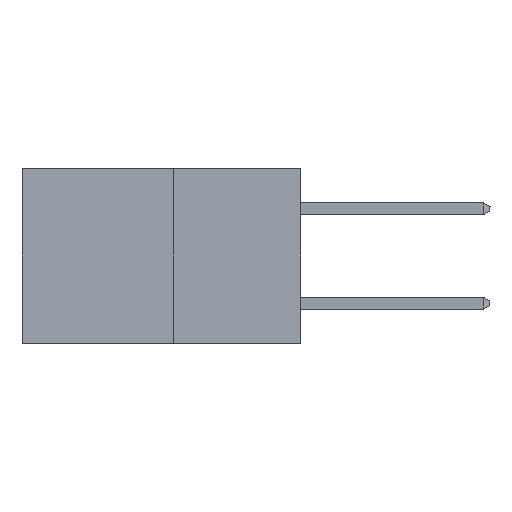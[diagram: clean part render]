
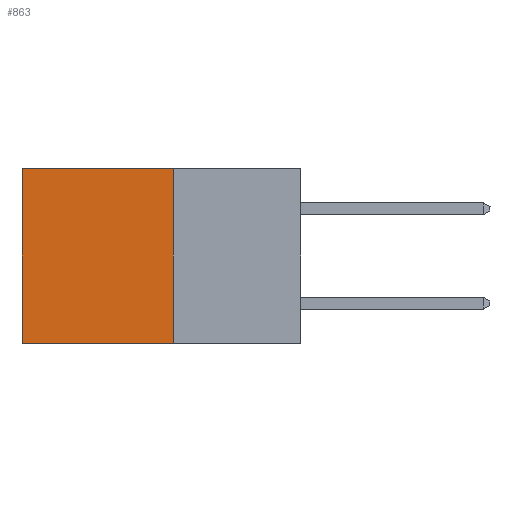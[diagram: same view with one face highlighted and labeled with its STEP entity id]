
A CAD part, left-side view. The second image highlights one B-rep face of the part: STEP entity #863.
In plain terms, the highlighted planar face has unit normal (-1, 0, 0).
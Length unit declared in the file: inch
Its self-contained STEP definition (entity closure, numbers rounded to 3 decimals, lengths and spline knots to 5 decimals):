
#84 = PLANE ( 'NONE',  #2871 ) ;
#150 = EDGE_CURVE ( 'NONE', #2724, #8112, #6001, .T. ) ;
#863 = ADVANCED_FACE ( 'NONE', ( #5290 ), #84, .F. ) ;
#902 = EDGE_CURVE ( 'NONE', #10497, #6457, #2334, .T. ) ;
#979 = ORIENTED_EDGE ( 'NONE', *, *, #902, .T. ) ;
#1040 = DIRECTION ( 'NONE',  ( 0., 0., -1. ) ) ;
#1282 = CARTESIAN_POINT ( 'NONE',  ( 0.277, 0.27, 0. ) ) ;
#2030 = EDGE_LOOP ( 'NONE', ( #979, #2833, #5757, #5247 ) ) ;
#2334 = LINE ( 'NONE', #10953, #6819 ) ;
#2363 = EDGE_CURVE ( 'NONE', #8112, #6457, #9028, .T. ) ;
#2724 = VERTEX_POINT ( 'NONE', #1282 ) ;
#2833 = ORIENTED_EDGE ( 'NONE', *, *, #2363, .F. ) ;
#2871 = AXIS2_PLACEMENT_3D ( 'NONE', #8211, #6450, #1040 ) ;
#3602 = EDGE_CURVE ( 'NONE', #2724, #10497, #7363, .T. ) ;
#3968 = CARTESIAN_POINT ( 'NONE',  ( 0.277, 0.27, -0.37 ) ) ;
#5178 = CARTESIAN_POINT ( 'NONE',  ( 0.277, 0.27, -0.37 ) ) ;
#5247 = ORIENTED_EDGE ( 'NONE', *, *, #3602, .T. ) ;
#5290 = FACE_OUTER_BOUND ( 'NONE', #2030, .T. ) ;
#5425 = CARTESIAN_POINT ( 'NONE',  ( 0.277, 0.27, -0.37 ) ) ;
#5757 = ORIENTED_EDGE ( 'NONE', *, *, #150, .F. ) ;
#6001 = LINE ( 'NONE', #3968, #7861 ) ;
#6045 = CARTESIAN_POINT ( 'NONE',  ( 0.277, 0.27, 0. ) ) ;
#6450 = DIRECTION ( 'NONE',  ( 1., 0., 0. ) ) ;
#6457 = VERTEX_POINT ( 'NONE', #6774 ) ;
#6608 = DIRECTION ( 'NONE',  ( 0., 0., -1. ) ) ;
#6637 = VECTOR ( 'NONE', #7957, 39.37008 ) ;
#6774 = CARTESIAN_POINT ( 'NONE',  ( 0.277, 0.59, -0.37 ) ) ;
#6819 = VECTOR ( 'NONE', #7472, 39.37008 ) ;
#7363 = LINE ( 'NONE', #6045, #9687 ) ;
#7472 = DIRECTION ( 'NONE',  ( 0., 0., -1. ) ) ;
#7861 = VECTOR ( 'NONE', #6608, 39.37008 ) ;
#7957 = DIRECTION ( 'NONE',  ( 0., 1., 0. ) ) ;
#8112 = VERTEX_POINT ( 'NONE', #5425 ) ;
#8211 = CARTESIAN_POINT ( 'NONE',  ( 0.277, 0.27, -0.37 ) ) ;
#9028 = LINE ( 'NONE', #5178, #6637 ) ;
#9687 = VECTOR ( 'NONE', #10475, 39.37008 ) ;
#10475 = DIRECTION ( 'NONE',  ( 0., 1., 0. ) ) ;
#10491 = CARTESIAN_POINT ( 'NONE',  ( 0.277, 0.59, 0. ) ) ;
#10497 = VERTEX_POINT ( 'NONE', #10491 ) ;
#10953 = CARTESIAN_POINT ( 'NONE',  ( 0.277, 0.59, -0.37 ) ) ;
